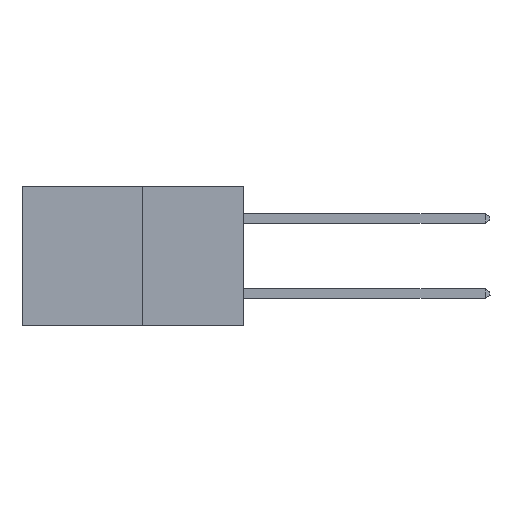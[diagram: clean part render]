
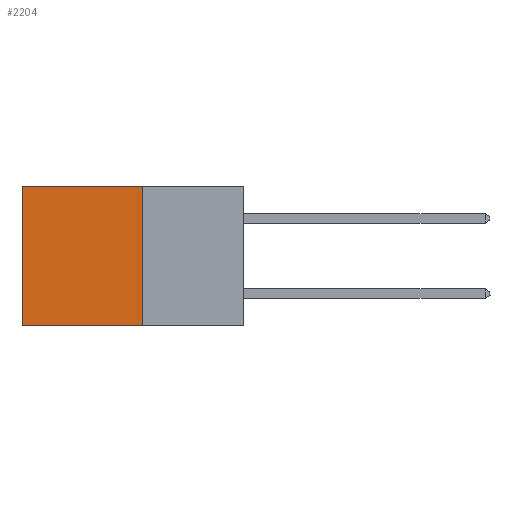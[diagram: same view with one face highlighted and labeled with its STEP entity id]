
A CAD part, left-side view. The second image highlights one B-rep face of the part: STEP entity #2204.
In plain terms, the highlighted planar face has unit normal (-1, 0, 0).
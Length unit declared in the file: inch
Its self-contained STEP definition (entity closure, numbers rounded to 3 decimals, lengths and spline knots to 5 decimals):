
#198 = EDGE_LOOP ( 'NONE', ( #605, #5536, #7986, #5741 ) ) ;
#513 = CARTESIAN_POINT ( 'NONE',  ( 0.277, 0.27, 0. ) ) ;
#605 = ORIENTED_EDGE ( 'NONE', *, *, #10856, .T. ) ;
#661 = DIRECTION ( 'NONE',  ( 0., 0., -1. ) ) ;
#664 = EDGE_CURVE ( 'NONE', #1962, #10538, #6636, .T. ) ;
#1464 = CARTESIAN_POINT ( 'NONE',  ( 0.277, 0.59, 0. ) ) ;
#1846 = DIRECTION ( 'NONE',  ( 0., 1., 0. ) ) ;
#1962 = VERTEX_POINT ( 'NONE', #4866 ) ;
#2204 = ADVANCED_FACE ( 'NONE', ( #4932 ), #4276, .F. ) ;
#2397 = LINE ( 'NONE', #9298, #10867 ) ;
#2558 = DIRECTION ( 'NONE',  ( 0., 0., -1. ) ) ;
#3002 = CARTESIAN_POINT ( 'NONE',  ( 0.277, 0.27, -0.37 ) ) ;
#3206 = EDGE_CURVE ( 'NONE', #10538, #3974, #2397, .T. ) ;
#3974 = VERTEX_POINT ( 'NONE', #10270 ) ;
#4276 = PLANE ( 'NONE',  #6610 ) ;
#4428 = VECTOR ( 'NONE', #661, 39.37008 ) ;
#4866 = CARTESIAN_POINT ( 'NONE',  ( 0.277, 0.27, 0. ) ) ;
#4932 = FACE_OUTER_BOUND ( 'NONE', #198, .T. ) ;
#5536 = ORIENTED_EDGE ( 'NONE', *, *, #3206, .F. ) ;
#5741 = ORIENTED_EDGE ( 'NONE', *, *, #8888, .T. ) ;
#5824 = DIRECTION ( 'NONE',  ( 0., 1., 0. ) ) ;
#6610 = AXIS2_PLACEMENT_3D ( 'NONE', #10561, #10556, #10491 ) ;
#6636 = LINE ( 'NONE', #10780, #4428 ) ;
#7986 = ORIENTED_EDGE ( 'NONE', *, *, #664, .F. ) ;
#8350 = CARTESIAN_POINT ( 'NONE',  ( 0.277, 0.59, -0.37 ) ) ;
#8587 = VECTOR ( 'NONE', #2558, 39.37008 ) ;
#8739 = VERTEX_POINT ( 'NONE', #1464 ) ;
#8888 = EDGE_CURVE ( 'NONE', #1962, #8739, #10022, .T. ) ;
#9298 = CARTESIAN_POINT ( 'NONE',  ( 0.277, 0.27, -0.37 ) ) ;
#9769 = VECTOR ( 'NONE', #5824, 39.37008 ) ;
#10022 = LINE ( 'NONE', #513, #9769 ) ;
#10270 = CARTESIAN_POINT ( 'NONE',  ( 0.277, 0.59, -0.37 ) ) ;
#10491 = DIRECTION ( 'NONE',  ( 0., 0., -1. ) ) ;
#10538 = VERTEX_POINT ( 'NONE', #3002 ) ;
#10556 = DIRECTION ( 'NONE',  ( 1., 0., 0. ) ) ;
#10561 = CARTESIAN_POINT ( 'NONE',  ( 0.277, 0.27, -0.37 ) ) ;
#10780 = CARTESIAN_POINT ( 'NONE',  ( 0.277, 0.27, -0.37 ) ) ;
#10856 = EDGE_CURVE ( 'NONE', #8739, #3974, #10961, .T. ) ;
#10867 = VECTOR ( 'NONE', #1846, 39.37008 ) ;
#10961 = LINE ( 'NONE', #8350, #8587 ) ;
